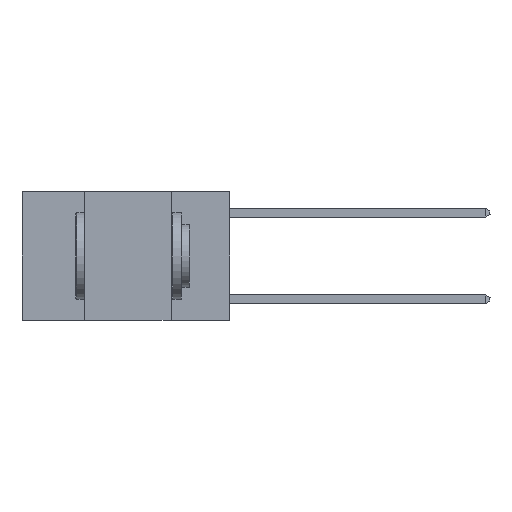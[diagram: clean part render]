
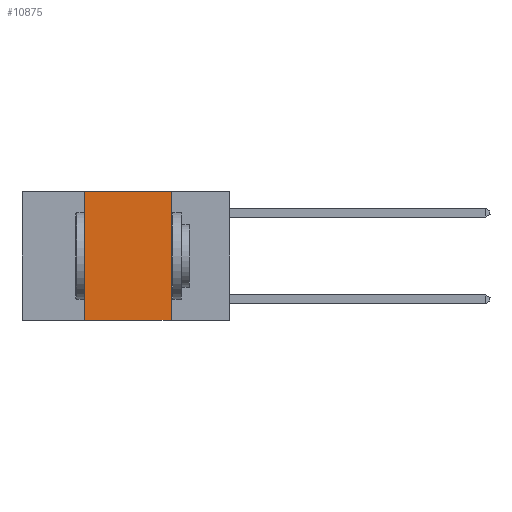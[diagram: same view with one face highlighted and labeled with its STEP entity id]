
A CAD part, left-side view. The second image highlights one B-rep face of the part: STEP entity #10875.
In plain terms, the highlighted planar face has unit normal (-1, 0, 0).
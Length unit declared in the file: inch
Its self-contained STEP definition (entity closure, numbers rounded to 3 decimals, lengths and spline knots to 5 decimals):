
#905 = ORIENTED_EDGE ( 'NONE', *, *, #16063, .F. ) ;
#1046 = DIRECTION ( 'NONE',  ( 0., 0., -1. ) ) ;
#1226 = LINE ( 'NONE', #3032, #5516 ) ;
#1436 = DIRECTION ( 'NONE',  ( 1., 0., 0. ) ) ;
#1571 = CARTESIAN_POINT ( 'NONE',  ( 0., 0.6, 0. ) ) ;
#3032 = CARTESIAN_POINT ( 'NONE',  ( 0., 0.6, -0.37 ) ) ;
#3374 = LINE ( 'NONE', #11002, #20982 ) ;
#5104 = CARTESIAN_POINT ( 'NONE',  ( 0., 0.17, 0. ) ) ;
#5210 = FACE_OUTER_BOUND ( 'NONE', #23572, .T. ) ;
#5516 = VECTOR ( 'NONE', #9122, 39.37008 ) ;
#7309 = LINE ( 'NONE', #5104, #16464 ) ;
#7548 = DIRECTION ( 'NONE',  ( 0., 0., -1. ) ) ;
#7613 = LINE ( 'NONE', #15882, #21322 ) ;
#7729 = CARTESIAN_POINT ( 'NONE',  ( 0., 0.17, 0. ) ) ;
#8098 = CARTESIAN_POINT ( 'NONE',  ( 0., 0.42, 0. ) ) ;
#9076 = ORIENTED_EDGE ( 'NONE', *, *, #12782, .F. ) ;
#9122 = DIRECTION ( 'NONE',  ( 0., -1., 0. ) ) ;
#9583 = CARTESIAN_POINT ( 'NONE',  ( 0., 0.17, -0.37 ) ) ;
#10325 = EDGE_CURVE ( 'NONE', #24367, #12364, #7309, .T. ) ;
#10875 = ADVANCED_FACE ( 'NONE', ( #5210 ), #16960, .F. ) ;
#11002 = CARTESIAN_POINT ( 'NONE',  ( 0., 0.6, 0. ) ) ;
#11072 = ORIENTED_EDGE ( 'NONE', *, *, #10325, .F. ) ;
#12364 = VERTEX_POINT ( 'NONE', #9583 ) ;
#12782 = EDGE_CURVE ( 'NONE', #20289, #13416, #7613, .T. ) ;
#13416 = VERTEX_POINT ( 'NONE', #8098 ) ;
#13459 = DIRECTION ( 'NONE',  ( 0., -1., 0. ) ) ;
#13480 = CARTESIAN_POINT ( 'NONE',  ( 0., 0.42, -0.37 ) ) ;
#14612 = AXIS2_PLACEMENT_3D ( 'NONE', #1571, #1436, #1046 ) ;
#15882 = CARTESIAN_POINT ( 'NONE',  ( 0., 0.42, 0. ) ) ;
#16063 = EDGE_CURVE ( 'NONE', #13416, #24367, #3374, .T. ) ;
#16464 = VECTOR ( 'NONE', #7548, 39.37008 ) ;
#16960 = PLANE ( 'NONE',  #14612 ) ;
#17969 = DIRECTION ( 'NONE',  ( 0., 0., 1. ) ) ;
#19810 = EDGE_CURVE ( 'NONE', #20289, #12364, #1226, .T. ) ;
#20289 = VERTEX_POINT ( 'NONE', #13480 ) ;
#20474 = ORIENTED_EDGE ( 'NONE', *, *, #19810, .T. ) ;
#20982 = VECTOR ( 'NONE', #13459, 39.37008 ) ;
#21322 = VECTOR ( 'NONE', #17969, 39.37008 ) ;
#23572 = EDGE_LOOP ( 'NONE', ( #11072, #905, #9076, #20474 ) ) ;
#24367 = VERTEX_POINT ( 'NONE', #7729 ) ;
